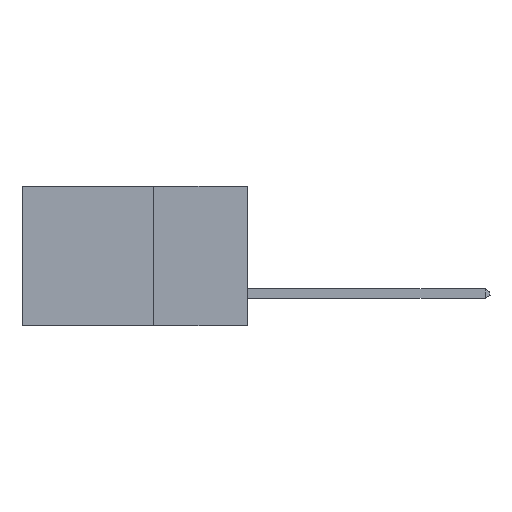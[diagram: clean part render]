
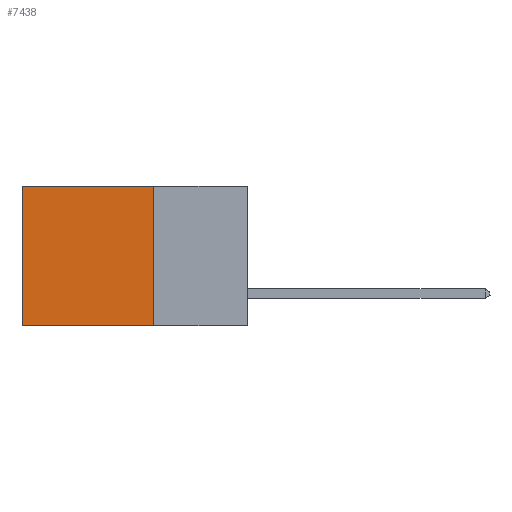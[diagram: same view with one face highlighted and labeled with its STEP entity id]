
A CAD part, left-side view. The second image highlights one B-rep face of the part: STEP entity #7438.
In plain terms, the highlighted planar face has unit normal (-1, 0, 0).
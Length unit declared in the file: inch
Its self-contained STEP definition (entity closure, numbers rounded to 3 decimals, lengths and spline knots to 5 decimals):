
#14 = VERTEX_POINT ( 'NONE', #1099 ) ;
#268 = VERTEX_POINT ( 'NONE', #7922 ) ;
#532 = LINE ( 'NONE', #1046, #1635 ) ;
#1046 = CARTESIAN_POINT ( 'NONE',  ( 0.298, 0.25, -0.37 ) ) ;
#1099 = CARTESIAN_POINT ( 'NONE',  ( 0.298, 0.6, 0. ) ) ;
#1635 = VECTOR ( 'NONE', #2635, 39.37008 ) ;
#1838 = FACE_OUTER_BOUND ( 'NONE', #7452, .T. ) ;
#1931 = ORIENTED_EDGE ( 'NONE', *, *, #5039, .F. ) ;
#1946 = CARTESIAN_POINT ( 'NONE',  ( 0.298, 0.25, 0. ) ) ;
#2107 = EDGE_CURVE ( 'NONE', #7778, #14, #4964, .T. ) ;
#2201 = DIRECTION ( 'NONE',  ( 0., 0., -1. ) ) ;
#2491 = VECTOR ( 'NONE', #2201, 39.37008 ) ;
#2635 = DIRECTION ( 'NONE',  ( 0., 1., 0. ) ) ;
#2850 = VECTOR ( 'NONE', #6262, 39.37008 ) ;
#3040 = CARTESIAN_POINT ( 'NONE',  ( 0.298, 0.25, 0. ) ) ;
#3204 = ORIENTED_EDGE ( 'NONE', *, *, #4249, .F. ) ;
#3629 = CARTESIAN_POINT ( 'NONE',  ( 0.298, 0.6, 0. ) ) ;
#3828 = AXIS2_PLACEMENT_3D ( 'NONE', #3040, #6219, #7024 ) ;
#4249 = EDGE_CURVE ( 'NONE', #7778, #8196, #5413, .T. ) ;
#4964 = LINE ( 'NONE', #10260, #2850 ) ;
#5039 = EDGE_CURVE ( 'NONE', #8196, #268, #532, .T. ) ;
#5413 = LINE ( 'NONE', #5892, #7935 ) ;
#5799 = ORIENTED_EDGE ( 'NONE', *, *, #6408, .T. ) ;
#5892 = CARTESIAN_POINT ( 'NONE',  ( 0.298, 0.25, 0. ) ) ;
#6219 = DIRECTION ( 'NONE',  ( 1., 0., 0. ) ) ;
#6262 = DIRECTION ( 'NONE',  ( 0., 1., 0. ) ) ;
#6408 = EDGE_CURVE ( 'NONE', #14, #268, #8407, .T. ) ;
#6867 = CARTESIAN_POINT ( 'NONE',  ( 0.298, 0.25, -0.37 ) ) ;
#7024 = DIRECTION ( 'NONE',  ( 0., 0., -1. ) ) ;
#7438 = ADVANCED_FACE ( 'NONE', ( #1838 ), #9455, .F. ) ;
#7452 = EDGE_LOOP ( 'NONE', ( #5799, #1931, #3204, #10101 ) ) ;
#7778 = VERTEX_POINT ( 'NONE', #1946 ) ;
#7922 = CARTESIAN_POINT ( 'NONE',  ( 0.298, 0.6, -0.37 ) ) ;
#7935 = VECTOR ( 'NONE', #9031, 39.37008 ) ;
#8196 = VERTEX_POINT ( 'NONE', #6867 ) ;
#8407 = LINE ( 'NONE', #3629, #2491 ) ;
#9031 = DIRECTION ( 'NONE',  ( 0., 0., -1. ) ) ;
#9455 = PLANE ( 'NONE',  #3828 ) ;
#10101 = ORIENTED_EDGE ( 'NONE', *, *, #2107, .T. ) ;
#10260 = CARTESIAN_POINT ( 'NONE',  ( 0.298, 0.25, 0. ) ) ;
